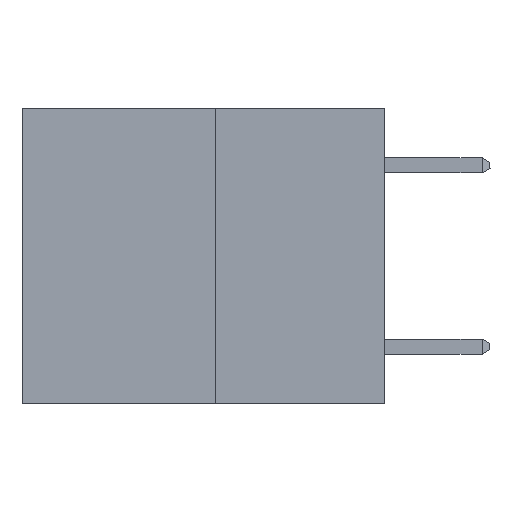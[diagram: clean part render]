
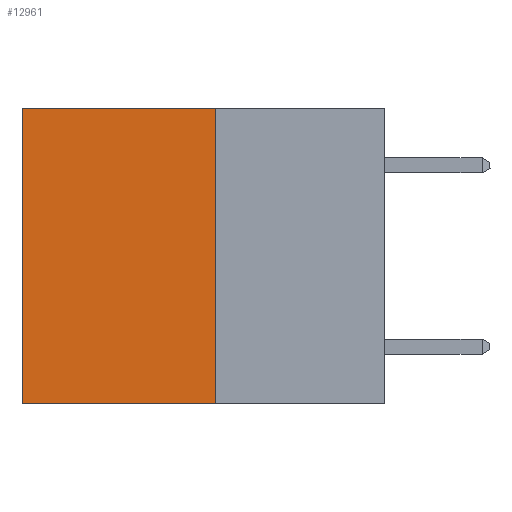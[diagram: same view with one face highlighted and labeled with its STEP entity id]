
A CAD part, left-side view. The second image highlights one B-rep face of the part: STEP entity #12961.
In plain terms, the highlighted planar face has unit normal (-1, 0, 0).
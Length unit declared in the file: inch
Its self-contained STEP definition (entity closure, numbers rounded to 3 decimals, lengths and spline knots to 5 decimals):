
#1557 = ORIENTED_EDGE ( 'NONE', *, *, #1640, .F. ) ;
#1640 = EDGE_CURVE ( 'NONE', #25000, #3489, #5458, .T. ) ;
#3489 = VERTEX_POINT ( 'NONE', #24609 ) ;
#3829 = LINE ( 'NONE', #7919, #11036 ) ;
#3991 = ORIENTED_EDGE ( 'NONE', *, *, #12822, .T. ) ;
#5458 = LINE ( 'NONE', #23206, #27628 ) ;
#6764 = LINE ( 'NONE', #15393, #25757 ) ;
#7919 = CARTESIAN_POINT ( 'NONE',  ( 0.3165, 0.28, 0. ) ) ;
#8726 = PLANE ( 'NONE',  #16556 ) ;
#8770 = EDGE_LOOP ( 'NONE', ( #20918, #1557, #11889, #3991 ) ) ;
#11036 = VECTOR ( 'NONE', #19558, 39.37008 ) ;
#11549 = EDGE_CURVE ( 'NONE', #29191, #25000, #6764, .T. ) ;
#11752 = CARTESIAN_POINT ( 'NONE',  ( 0.3165, 0.28, -0.49 ) ) ;
#11889 = ORIENTED_EDGE ( 'NONE', *, *, #11549, .F. ) ;
#12507 = CARTESIAN_POINT ( 'NONE',  ( 0.3165, 0.28, -0.49 ) ) ;
#12822 = EDGE_CURVE ( 'NONE', #29191, #19055, #3829, .T. ) ;
#12961 = ADVANCED_FACE ( 'NONE', ( #19595 ), #8726, .F. ) ;
#14025 = DIRECTION ( 'NONE',  ( 1., 0., 0. ) ) ;
#15393 = CARTESIAN_POINT ( 'NONE',  ( 0.3165, 0.28, -0.49 ) ) ;
#15662 = CARTESIAN_POINT ( 'NONE',  ( 0.3165, 0.6, 0. ) ) ;
#16556 = AXIS2_PLACEMENT_3D ( 'NONE', #11752, #14025, #18656 ) ;
#16969 = EDGE_CURVE ( 'NONE', #19055, #3489, #24735, .T. ) ;
#18656 = DIRECTION ( 'NONE',  ( 0., 0., -1. ) ) ;
#19055 = VERTEX_POINT ( 'NONE', #15662 ) ;
#19558 = DIRECTION ( 'NONE',  ( 0., 1., 0. ) ) ;
#19595 = FACE_OUTER_BOUND ( 'NONE', #8770, .T. ) ;
#20700 = DIRECTION ( 'NONE',  ( 0., 1., 0. ) ) ;
#20918 = ORIENTED_EDGE ( 'NONE', *, *, #16969, .T. ) ;
#22360 = CARTESIAN_POINT ( 'NONE',  ( 0.3165, 0.6, -0.49 ) ) ;
#23206 = CARTESIAN_POINT ( 'NONE',  ( 0.3165, 0.28, -0.49 ) ) ;
#24609 = CARTESIAN_POINT ( 'NONE',  ( 0.3165, 0.6, -0.49 ) ) ;
#24735 = LINE ( 'NONE', #22360, #26542 ) ;
#24976 = CARTESIAN_POINT ( 'NONE',  ( 0.3165, 0.28, 0. ) ) ;
#25000 = VERTEX_POINT ( 'NONE', #12507 ) ;
#25757 = VECTOR ( 'NONE', #29305, 39.37008 ) ;
#26542 = VECTOR ( 'NONE', #26971, 39.37008 ) ;
#26971 = DIRECTION ( 'NONE',  ( 0., 0., -1. ) ) ;
#27628 = VECTOR ( 'NONE', #20700, 39.37008 ) ;
#29191 = VERTEX_POINT ( 'NONE', #24976 ) ;
#29305 = DIRECTION ( 'NONE',  ( 0., 0., -1. ) ) ;
